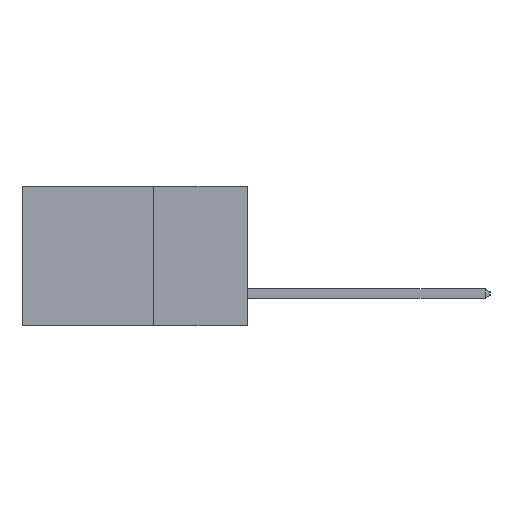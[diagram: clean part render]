
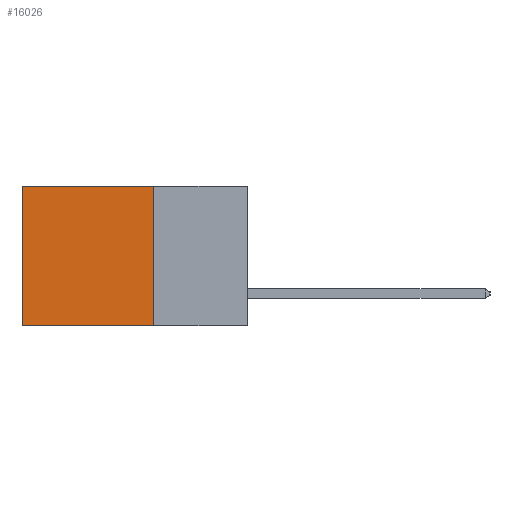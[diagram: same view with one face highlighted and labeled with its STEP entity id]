
A CAD part, left-side view. The second image highlights one B-rep face of the part: STEP entity #16026.
In plain terms, the highlighted planar face has unit normal (-1, 0, 0).
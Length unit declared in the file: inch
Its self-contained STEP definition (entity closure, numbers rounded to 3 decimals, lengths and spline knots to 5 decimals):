
#1873 = VECTOR ( 'NONE', #16440, 39.37008 ) ;
#3415 = CARTESIAN_POINT ( 'NONE',  ( 0.298, 0.25, 0. ) ) ;
#4048 = DIRECTION ( 'NONE',  ( 0., 0., -1. ) ) ;
#5444 = CARTESIAN_POINT ( 'NONE',  ( 0.298, 0.25, 0. ) ) ;
#6716 = VERTEX_POINT ( 'NONE', #3415 ) ;
#8764 = VECTOR ( 'NONE', #11590, 39.37008 ) ;
#10598 = AXIS2_PLACEMENT_3D ( 'NONE', #25746, #27969, #14647 ) ;
#11017 = CARTESIAN_POINT ( 'NONE',  ( 0.298, 0.6, -0.37 ) ) ;
#11065 = LINE ( 'NONE', #19621, #27444 ) ;
#11590 = DIRECTION ( 'NONE',  ( 0., 1., 0. ) ) ;
#13084 = VERTEX_POINT ( 'NONE', #19595 ) ;
#13489 = EDGE_LOOP ( 'NONE', ( #15643, #23506, #23400, #14416 ) ) ;
#13638 = LINE ( 'NONE', #16335, #1873 ) ;
#14416 = ORIENTED_EDGE ( 'NONE', *, *, #20288, .T. ) ;
#14451 = CARTESIAN_POINT ( 'NONE',  ( 0.298, 0.6, 0. ) ) ;
#14647 = DIRECTION ( 'NONE',  ( 0., 0., -1. ) ) ;
#14709 = LINE ( 'NONE', #18266, #8764 ) ;
#15643 = ORIENTED_EDGE ( 'NONE', *, *, #19222, .T. ) ;
#16026 = ADVANCED_FACE ( 'NONE', ( #23292 ), #23551, .F. ) ;
#16264 = VERTEX_POINT ( 'NONE', #11017 ) ;
#16335 = CARTESIAN_POINT ( 'NONE',  ( 0.298, 0.25, -0.37 ) ) ;
#16440 = DIRECTION ( 'NONE',  ( 0., 1., 0. ) ) ;
#18266 = CARTESIAN_POINT ( 'NONE',  ( 0.298, 0.25, 0. ) ) ;
#19222 = EDGE_CURVE ( 'NONE', #25663, #16264, #11065, .T. ) ;
#19595 = CARTESIAN_POINT ( 'NONE',  ( 0.298, 0.25, -0.37 ) ) ;
#19621 = CARTESIAN_POINT ( 'NONE',  ( 0.298, 0.6, 0. ) ) ;
#20288 = EDGE_CURVE ( 'NONE', #6716, #25663, #14709, .T. ) ;
#21005 = EDGE_CURVE ( 'NONE', #13084, #16264, #13638, .T. ) ;
#22590 = VECTOR ( 'NONE', #25494, 39.37008 ) ;
#22920 = EDGE_CURVE ( 'NONE', #6716, #13084, #28447, .T. ) ;
#23292 = FACE_OUTER_BOUND ( 'NONE', #13489, .T. ) ;
#23400 = ORIENTED_EDGE ( 'NONE', *, *, #22920, .F. ) ;
#23506 = ORIENTED_EDGE ( 'NONE', *, *, #21005, .F. ) ;
#23551 = PLANE ( 'NONE',  #10598 ) ;
#25494 = DIRECTION ( 'NONE',  ( 0., 0., -1. ) ) ;
#25663 = VERTEX_POINT ( 'NONE', #14451 ) ;
#25746 = CARTESIAN_POINT ( 'NONE',  ( 0.298, 0.25, 0. ) ) ;
#27444 = VECTOR ( 'NONE', #4048, 39.37008 ) ;
#27969 = DIRECTION ( 'NONE',  ( 1., 0., 0. ) ) ;
#28447 = LINE ( 'NONE', #5444, #22590 ) ;
